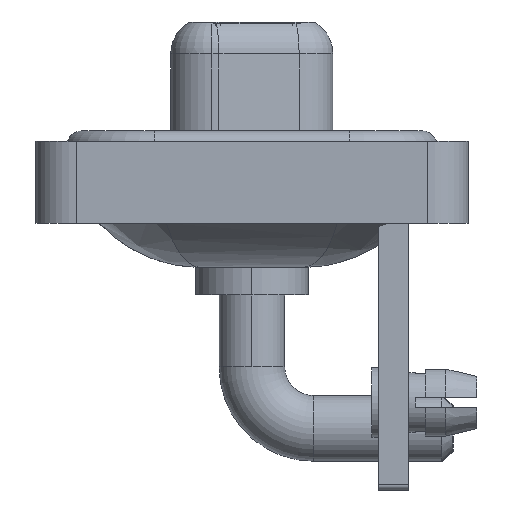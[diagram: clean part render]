
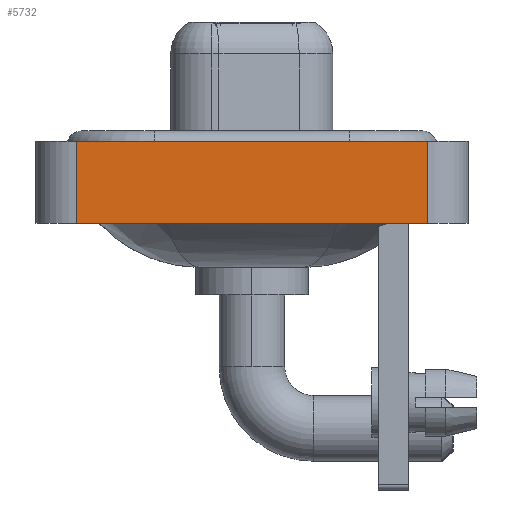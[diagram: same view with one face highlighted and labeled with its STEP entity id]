
A CAD part, left-side view. The second image highlights one B-rep face of the part: STEP entity #5732.
In plain terms, the highlighted planar face has unit normal (-1, 0, 0).
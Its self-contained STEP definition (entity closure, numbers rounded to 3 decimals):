
#33 = DIRECTION ( 'NONE',  ( 0., -1., 0. ) ) ;
#102 = EDGE_CURVE ( 'NONE', #15086, #5828, #7590, .T. ) ;
#251 = CARTESIAN_POINT ( 'NONE',  ( -7.25, -8.55, -3.6 ) ) ;
#1494 = CARTESIAN_POINT ( 'NONE',  ( -7.25, -8.55, -3.6 ) ) ;
#3733 = FACE_OUTER_BOUND ( 'NONE', #9741, .T. ) ;
#4014 = EDGE_CURVE ( 'NONE', #15086, #9413, #10555, .T. ) ;
#4227 = DIRECTION ( 'NONE',  ( 0., 0., 1. ) ) ;
#5595 = CARTESIAN_POINT ( 'NONE',  ( -7.25, -8.55, -3.6 ) ) ;
#5732 = ADVANCED_FACE ( 'NONE', ( #3733 ), #11349, .T. ) ;
#5755 = ORIENTED_EDGE ( 'NONE', *, *, #4014, .F. ) ;
#5828 = VERTEX_POINT ( 'NONE', #251 ) ;
#5852 = VECTOR ( 'NONE', #15259, 1000. ) ;
#5980 = CARTESIAN_POINT ( 'NONE',  ( -7.25, 8.55, 0.4 ) ) ;
#6573 = ORIENTED_EDGE ( 'NONE', *, *, #102, .T. ) ;
#7243 = EDGE_CURVE ( 'NONE', #9413, #16830, #16399, .T. ) ;
#7590 = LINE ( 'NONE', #1494, #12812 ) ;
#7731 = CARTESIAN_POINT ( 'NONE',  ( -7.25, 8.55, -3.6 ) ) ;
#7799 = ORIENTED_EDGE ( 'NONE', *, *, #7243, .F. ) ;
#8897 = EDGE_CURVE ( 'NONE', #5828, #16830, #17677, .T. ) ;
#9413 = VERTEX_POINT ( 'NONE', #5980 ) ;
#9642 = VECTOR ( 'NONE', #4227, 1000. ) ;
#9741 = EDGE_LOOP ( 'NONE', ( #14481, #7799, #5755, #6573 ) ) ;
#10555 = LINE ( 'NONE', #7731, #5852 ) ;
#11349 = PLANE ( 'NONE',  #12142 ) ;
#11544 = DIRECTION ( 'NONE',  ( -1., 0., 0. ) ) ;
#12142 = AXIS2_PLACEMENT_3D ( 'NONE', #5595, #11544, #17364 ) ;
#12424 = CARTESIAN_POINT ( 'NONE',  ( -7.25, 8.55, -3.6 ) ) ;
#12812 = VECTOR ( 'NONE', #33, 1000. ) ;
#14481 = ORIENTED_EDGE ( 'NONE', *, *, #8897, .T. ) ;
#14818 = DIRECTION ( 'NONE',  ( 0., -1., 0. ) ) ;
#15086 = VERTEX_POINT ( 'NONE', #12424 ) ;
#15259 = DIRECTION ( 'NONE',  ( 0., 0., 1. ) ) ;
#15958 = VECTOR ( 'NONE', #14818, 1000. ) ;
#16061 = CARTESIAN_POINT ( 'NONE',  ( -7.25, -8.55, 0.4 ) ) ;
#16399 = LINE ( 'NONE', #18091, #15958 ) ;
#16830 = VERTEX_POINT ( 'NONE', #16061 ) ;
#17364 = DIRECTION ( 'NONE',  ( 0., 0., 1. ) ) ;
#17677 = LINE ( 'NONE', #17981, #9642 ) ;
#17981 = CARTESIAN_POINT ( 'NONE',  ( -7.25, -8.55, -3.6 ) ) ;
#18091 = CARTESIAN_POINT ( 'NONE',  ( -7.25, -8.55, 0.4 ) ) ;
